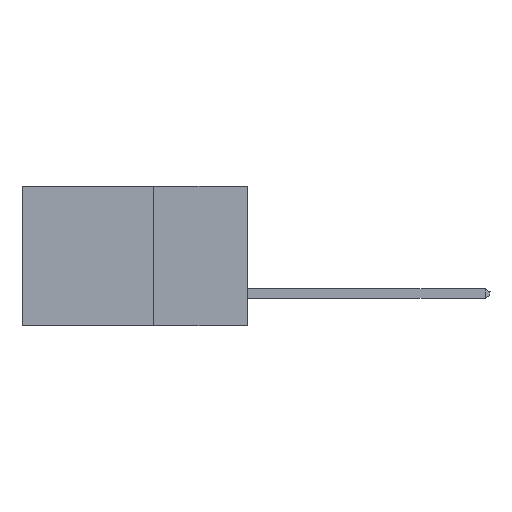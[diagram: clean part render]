
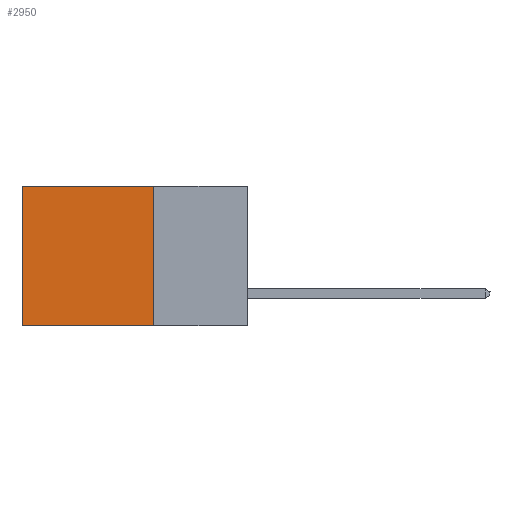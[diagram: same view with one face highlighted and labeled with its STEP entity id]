
A CAD part, left-side view. The second image highlights one B-rep face of the part: STEP entity #2950.
In plain terms, the highlighted planar face has unit normal (-1, 0, 0).
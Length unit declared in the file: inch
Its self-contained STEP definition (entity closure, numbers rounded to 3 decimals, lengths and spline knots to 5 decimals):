
#1021 = CARTESIAN_POINT ( 'NONE',  ( 0.2615, 0.6, -0.37 ) ) ;
#1152 = LINE ( 'NONE', #11667, #5172 ) ;
#1239 = FACE_OUTER_BOUND ( 'NONE', #4296, .T. ) ;
#1410 = CARTESIAN_POINT ( 'NONE',  ( 0.2615, 0.25, 0. ) ) ;
#1570 = DIRECTION ( 'NONE',  ( 0., 1., 0. ) ) ;
#1637 = ORIENTED_EDGE ( 'NONE', *, *, #12273, .T. ) ;
#2805 = VERTEX_POINT ( 'NONE', #14338 ) ;
#2950 = ADVANCED_FACE ( 'NONE', ( #1239 ), #5833, .F. ) ;
#2997 = ORIENTED_EDGE ( 'NONE', *, *, #7681, .F. ) ;
#3398 = CARTESIAN_POINT ( 'NONE',  ( 0.2615, 0.25, -0.37 ) ) ;
#3666 = VERTEX_POINT ( 'NONE', #1410 ) ;
#3999 = VERTEX_POINT ( 'NONE', #1021 ) ;
#4296 = EDGE_LOOP ( 'NONE', ( #1637, #2997, #14342, #11683 ) ) ;
#5172 = VECTOR ( 'NONE', #7221, 39.37008 ) ;
#5339 = VECTOR ( 'NONE', #1570, 39.37008 ) ;
#5355 = CARTESIAN_POINT ( 'NONE',  ( 0.2615, 0.6, 0. ) ) ;
#5688 = CARTESIAN_POINT ( 'NONE',  ( 0.2615, 0.25, -0.37 ) ) ;
#5833 = PLANE ( 'NONE',  #6823 ) ;
#6823 = AXIS2_PLACEMENT_3D ( 'NONE', #5688, #10191, #10334 ) ;
#6828 = VECTOR ( 'NONE', #7081, 39.37008 ) ;
#7081 = DIRECTION ( 'NONE',  ( 0., 0., -1. ) ) ;
#7199 = CARTESIAN_POINT ( 'NONE',  ( 0.2615, 0.25, 0. ) ) ;
#7221 = DIRECTION ( 'NONE',  ( 0., 0., -1. ) ) ;
#7681 = EDGE_CURVE ( 'NONE', #2805, #3999, #10981, .T. ) ;
#7925 = DIRECTION ( 'NONE',  ( 0., 1., 0. ) ) ;
#8619 = EDGE_CURVE ( 'NONE', #3666, #11615, #12728, .T. ) ;
#10191 = DIRECTION ( 'NONE',  ( 1., 0., 0. ) ) ;
#10334 = DIRECTION ( 'NONE',  ( 0., 0., -1. ) ) ;
#10981 = LINE ( 'NONE', #3398, #10991 ) ;
#10991 = VECTOR ( 'NONE', #7925, 39.37008 ) ;
#11374 = LINE ( 'NONE', #12536, #6828 ) ;
#11615 = VERTEX_POINT ( 'NONE', #5355 ) ;
#11667 = CARTESIAN_POINT ( 'NONE',  ( 0.2615, 0.6, -0.37 ) ) ;
#11683 = ORIENTED_EDGE ( 'NONE', *, *, #8619, .T. ) ;
#12201 = EDGE_CURVE ( 'NONE', #3666, #2805, #11374, .T. ) ;
#12273 = EDGE_CURVE ( 'NONE', #11615, #3999, #1152, .T. ) ;
#12536 = CARTESIAN_POINT ( 'NONE',  ( 0.2615, 0.25, -0.37 ) ) ;
#12728 = LINE ( 'NONE', #7199, #5339 ) ;
#14338 = CARTESIAN_POINT ( 'NONE',  ( 0.2615, 0.25, -0.37 ) ) ;
#14342 = ORIENTED_EDGE ( 'NONE', *, *, #12201, .F. ) ;
